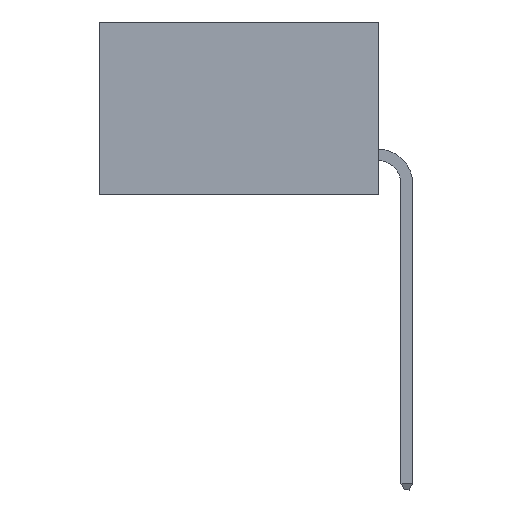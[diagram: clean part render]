
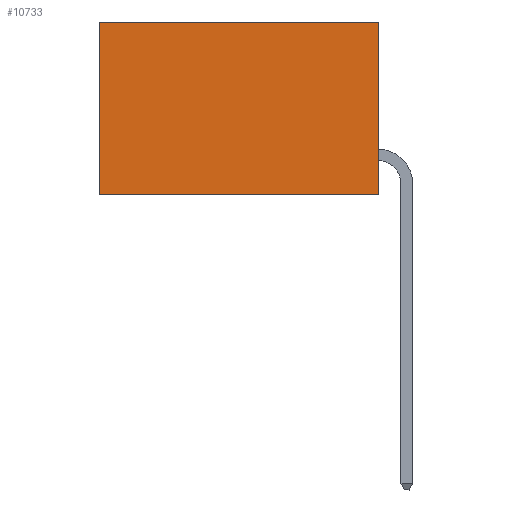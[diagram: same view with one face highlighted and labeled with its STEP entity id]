
A CAD part, left-side view. The second image highlights one B-rep face of the part: STEP entity #10733.
In plain terms, the highlighted planar face has unit normal (-1, 0, 0).
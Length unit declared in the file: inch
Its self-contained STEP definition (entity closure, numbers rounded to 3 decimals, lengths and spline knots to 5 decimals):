
#763 = CARTESIAN_POINT ( 'NONE',  ( 0.298, 0., 0. ) ) ;
#861 = ORIENTED_EDGE ( 'NONE', *, *, #19233, .F. ) ;
#3789 = ORIENTED_EDGE ( 'NONE', *, *, #22786, .T. ) ;
#3857 = EDGE_CURVE ( 'NONE', #7340, #23620, #4159, .T. ) ;
#4130 = VECTOR ( 'NONE', #17455, 39.37008 ) ;
#4159 = LINE ( 'NONE', #763, #22314 ) ;
#4270 = CARTESIAN_POINT ( 'NONE',  ( 0.298, 0.6, 0. ) ) ;
#4341 = EDGE_LOOP ( 'NONE', ( #3789, #861, #7437, #5141 ) ) ;
#5141 = ORIENTED_EDGE ( 'NONE', *, *, #3857, .T. ) ;
#5598 = DIRECTION ( 'NONE',  ( 0., 0., -1. ) ) ;
#6709 = CARTESIAN_POINT ( 'NONE',  ( 0.298, 0.6, -0.37 ) ) ;
#7340 = VERTEX_POINT ( 'NONE', #17085 ) ;
#7437 = ORIENTED_EDGE ( 'NONE', *, *, #9121, .F. ) ;
#8388 = PLANE ( 'NONE',  #23866 ) ;
#8849 = DIRECTION ( 'NONE',  ( 0., 1., 0. ) ) ;
#9121 = EDGE_CURVE ( 'NONE', #7340, #19845, #17890, .T. ) ;
#9710 = LINE ( 'NONE', #18329, #10292 ) ;
#10292 = VECTOR ( 'NONE', #8849, 39.37008 ) ;
#10733 = ADVANCED_FACE ( 'NONE', ( #12780 ), #8388, .F. ) ;
#11298 = CARTESIAN_POINT ( 'NONE',  ( 0.298, 0., -0.37 ) ) ;
#12042 = DIRECTION ( 'NONE',  ( 0., 1., 0. ) ) ;
#12780 = FACE_OUTER_BOUND ( 'NONE', #4341, .T. ) ;
#13773 = CARTESIAN_POINT ( 'NONE',  ( 0.298, 0., 0. ) ) ;
#14898 = VECTOR ( 'NONE', #5598, 39.37008 ) ;
#16732 = CARTESIAN_POINT ( 'NONE',  ( 0.298, 0.6, 0. ) ) ;
#17085 = CARTESIAN_POINT ( 'NONE',  ( 0.298, 0., 0. ) ) ;
#17455 = DIRECTION ( 'NONE',  ( 0., 0., -1. ) ) ;
#17890 = LINE ( 'NONE', #13773, #4130 ) ;
#18271 = DIRECTION ( 'NONE',  ( 0., 0., -1. ) ) ;
#18329 = CARTESIAN_POINT ( 'NONE',  ( 0.298, 0., -0.37 ) ) ;
#19233 = EDGE_CURVE ( 'NONE', #19845, #23763, #9710, .T. ) ;
#19288 = LINE ( 'NONE', #16732, #14898 ) ;
#19651 = CARTESIAN_POINT ( 'NONE',  ( 0.298, 0., 0. ) ) ;
#19845 = VERTEX_POINT ( 'NONE', #11298 ) ;
#22314 = VECTOR ( 'NONE', #12042, 39.37008 ) ;
#22786 = EDGE_CURVE ( 'NONE', #23620, #23763, #19288, .T. ) ;
#23620 = VERTEX_POINT ( 'NONE', #4270 ) ;
#23763 = VERTEX_POINT ( 'NONE', #6709 ) ;
#23866 = AXIS2_PLACEMENT_3D ( 'NONE', #19651, #24015, #18271 ) ;
#24015 = DIRECTION ( 'NONE',  ( 1., 0., 0. ) ) ;
